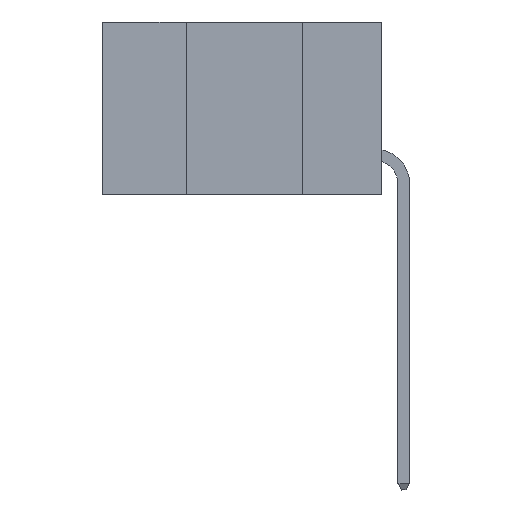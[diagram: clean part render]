
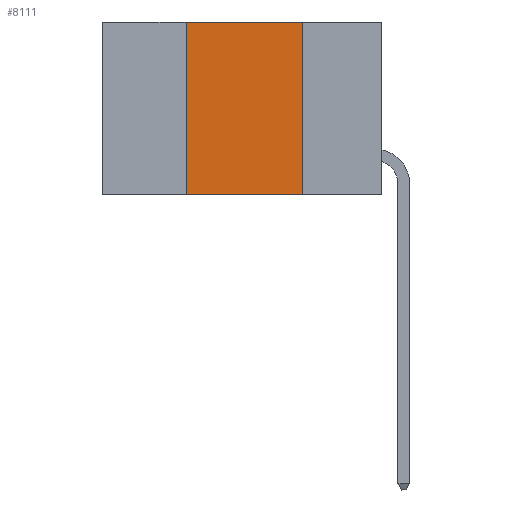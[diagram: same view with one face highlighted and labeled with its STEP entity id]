
A CAD part, left-side view. The second image highlights one B-rep face of the part: STEP entity #8111.
In plain terms, the highlighted planar face has unit normal (-1, 0, 0).
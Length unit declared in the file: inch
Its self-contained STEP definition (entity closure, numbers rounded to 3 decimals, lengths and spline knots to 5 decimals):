
#334 = LINE ( 'NONE', #7395, #9182 ) ;
#2619 = LINE ( 'NONE', #18809, #14973 ) ;
#2683 = CARTESIAN_POINT ( 'NONE',  ( 0., 0.42, -0.37 ) ) ;
#5055 = VERTEX_POINT ( 'NONE', #2683 ) ;
#5256 = EDGE_CURVE ( 'NONE', #20672, #15264, #2619, .T. ) ;
#5302 = DIRECTION ( 'NONE',  ( 1., 0., 0. ) ) ;
#6909 = LINE ( 'NONE', #14835, #21628 ) ;
#7322 = DIRECTION ( 'NONE',  ( 0., 0., 1. ) ) ;
#7395 = CARTESIAN_POINT ( 'NONE',  ( 0., 0.42, 0. ) ) ;
#8111 = ADVANCED_FACE ( 'NONE', ( #15955 ), #24321, .F. ) ;
#9182 = VECTOR ( 'NONE', #7322, 39.37008 ) ;
#9313 = DIRECTION ( 'NONE',  ( 0., 0., -1. ) ) ;
#9457 = ORIENTED_EDGE ( 'NONE', *, *, #23805, .F. ) ;
#9852 = EDGE_CURVE ( 'NONE', #5055, #11386, #14423, .T. ) ;
#11234 = AXIS2_PLACEMENT_3D ( 'NONE', #16455, #5302, #9313 ) ;
#11386 = VERTEX_POINT ( 'NONE', #16866 ) ;
#11463 = VECTOR ( 'NONE', #15561, 39.37008 ) ;
#11778 = CARTESIAN_POINT ( 'NONE',  ( 0., 0.6, -0.37 ) ) ;
#14423 = LINE ( 'NONE', #11778, #11463 ) ;
#14835 = CARTESIAN_POINT ( 'NONE',  ( 0., 0.17, 0. ) ) ;
#14973 = VECTOR ( 'NONE', #21770, 39.37008 ) ;
#15264 = VERTEX_POINT ( 'NONE', #21072 ) ;
#15561 = DIRECTION ( 'NONE',  ( 0., -1., 0. ) ) ;
#15668 = EDGE_CURVE ( 'NONE', #15264, #11386, #6909, .T. ) ;
#15955 = FACE_OUTER_BOUND ( 'NONE', #21866, .T. ) ;
#16455 = CARTESIAN_POINT ( 'NONE',  ( 0., 0.6, 0. ) ) ;
#16866 = CARTESIAN_POINT ( 'NONE',  ( 0., 0.17, -0.37 ) ) ;
#17161 = CARTESIAN_POINT ( 'NONE',  ( 0., 0.42, 0. ) ) ;
#17343 = DIRECTION ( 'NONE',  ( 0., 0., -1. ) ) ;
#18400 = ORIENTED_EDGE ( 'NONE', *, *, #9852, .T. ) ;
#18809 = CARTESIAN_POINT ( 'NONE',  ( 0., 0.6, 0. ) ) ;
#18840 = ORIENTED_EDGE ( 'NONE', *, *, #15668, .F. ) ;
#20672 = VERTEX_POINT ( 'NONE', #17161 ) ;
#21072 = CARTESIAN_POINT ( 'NONE',  ( 0., 0.17, 0. ) ) ;
#21627 = ORIENTED_EDGE ( 'NONE', *, *, #5256, .F. ) ;
#21628 = VECTOR ( 'NONE', #17343, 39.37008 ) ;
#21770 = DIRECTION ( 'NONE',  ( 0., -1., 0. ) ) ;
#21866 = EDGE_LOOP ( 'NONE', ( #18840, #21627, #9457, #18400 ) ) ;
#23805 = EDGE_CURVE ( 'NONE', #5055, #20672, #334, .T. ) ;
#24321 = PLANE ( 'NONE',  #11234 ) ;
